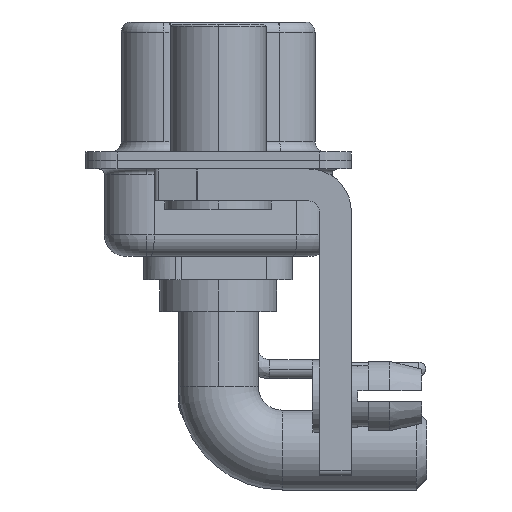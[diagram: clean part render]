
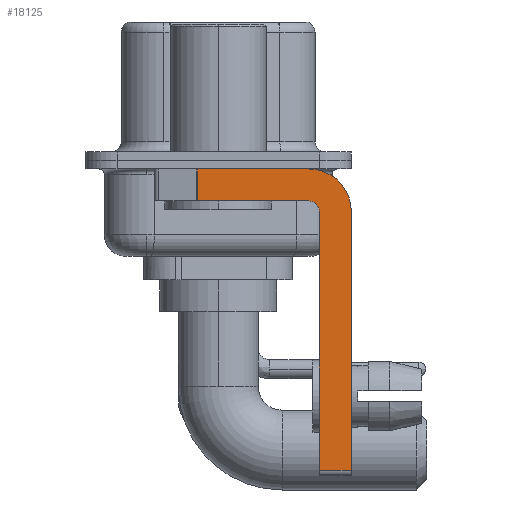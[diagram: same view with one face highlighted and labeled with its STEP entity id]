
A CAD part, left-side view. The second image highlights one B-rep face of the part: STEP entity #18125.
In plain terms, the highlighted planar face has unit normal (-1, 0, 0).
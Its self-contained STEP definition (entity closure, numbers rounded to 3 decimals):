
#287 = VERTEX_POINT ( 'NONE', #3551 ) ;
#379 = ORIENTED_EDGE ( 'NONE', *, *, #6843, .F. ) ;
#879 = DIRECTION ( 'NONE',  ( 0., 1., 0. ) ) ;
#1448 = EDGE_CURVE ( 'NONE', #28031, #14487, #7730, .T. ) ;
#1496 = CARTESIAN_POINT ( 'NONE',  ( -2.9, -4.25, -2.4 ) ) ;
#1642 = DIRECTION ( 'NONE',  ( 1., 0., 0. ) ) ;
#2060 = ORIENTED_EDGE ( 'NONE', *, *, #16158, .F. ) ;
#2559 = CARTESIAN_POINT ( 'NONE',  ( -2.9, 3., -0.4 ) ) ;
#3353 = EDGE_CURVE ( 'NONE', #16986, #287, #12311, .T. ) ;
#3551 = CARTESIAN_POINT ( 'NONE',  ( -2.9, -4.25, -1.9 ) ) ;
#4615 = VERTEX_POINT ( 'NONE', #22321 ) ;
#6075 = CARTESIAN_POINT ( 'NONE',  ( -2.9, -4.25, -0.4 ) ) ;
#6263 = LINE ( 'NONE', #14926, #11368 ) ;
#6843 = EDGE_CURVE ( 'NONE', #4615, #16986, #25310, .T. ) ;
#7092 = EDGE_CURVE ( 'NONE', #287, #12304, #11793, .T. ) ;
#7130 = CARTESIAN_POINT ( 'NONE',  ( -2.9, -4.25, -1.9 ) ) ;
#7249 = ORIENTED_EDGE ( 'NONE', *, *, #1448, .F. ) ;
#7374 = CARTESIAN_POINT ( 'NONE',  ( -2.9, -6.25, -2.4 ) ) ;
#7390 = CARTESIAN_POINT ( 'NONE',  ( -2.9, -4.25, -2.4 ) ) ;
#7487 = VECTOR ( 'NONE', #20185, 1000. ) ;
#7683 = VECTOR ( 'NONE', #21189, 1000. ) ;
#7730 = CIRCLE ( 'NONE', #23120, 2. ) ;
#7964 = DIRECTION ( 'NONE',  ( 0., 0., -1. ) ) ;
#8026 = DIRECTION ( 'NONE',  ( 0., 0., -1. ) ) ;
#8155 = ORIENTED_EDGE ( 'NONE', *, *, #24851, .F. ) ;
#8399 = DIRECTION ( 'NONE',  ( -1., 0., 0. ) ) ;
#9856 = EDGE_CURVE ( 'NONE', #27472, #12304, #6263, .T. ) ;
#11368 = VECTOR ( 'NONE', #7964, 1000. ) ;
#11793 = LINE ( 'NONE', #7130, #19446 ) ;
#12195 = LINE ( 'NONE', #7374, #16319 ) ;
#12304 = VERTEX_POINT ( 'NONE', #23825 ) ;
#12311 = CIRCLE ( 'NONE', #25896, 0.5 ) ;
#13154 = ORIENTED_EDGE ( 'NONE', *, *, #9856, .T. ) ;
#13364 = ORIENTED_EDGE ( 'NONE', *, *, #18329, .T. ) ;
#13800 = CARTESIAN_POINT ( 'NONE',  ( -2.9, -6.25, -2.4 ) ) ;
#13816 = CARTESIAN_POINT ( 'NONE',  ( -2.9, -4.25, -14.55 ) ) ;
#14419 = FACE_OUTER_BOUND ( 'NONE', #21427, .T. ) ;
#14487 = VERTEX_POINT ( 'NONE', #13800 ) ;
#14926 = CARTESIAN_POINT ( 'NONE',  ( -2.9, 0.978, -1.9 ) ) ;
#15188 = LINE ( 'NONE', #2559, #20633 ) ;
#16158 = EDGE_CURVE ( 'NONE', #27472, #28031, #15188, .T. ) ;
#16173 = CARTESIAN_POINT ( 'NONE',  ( -2.9, -6.25, -14.55 ) ) ;
#16319 = VECTOR ( 'NONE', #20415, 1000. ) ;
#16986 = VERTEX_POINT ( 'NONE', #25186 ) ;
#17198 = CARTESIAN_POINT ( 'NONE',  ( -2.9, -4.25, -2.4 ) ) ;
#18125 = ADVANCED_FACE ( 'NONE', ( #14419 ), #27313, .F. ) ;
#18329 = EDGE_CURVE ( 'NONE', #4615, #24887, #22036, .T. ) ;
#18885 = DIRECTION ( 'NONE',  ( 0., 0., 1. ) ) ;
#19446 = VECTOR ( 'NONE', #879, 1000. ) ;
#19543 = ORIENTED_EDGE ( 'NONE', *, *, #7092, .F. ) ;
#20011 = DIRECTION ( 'NONE',  ( 1., 0., 0. ) ) ;
#20185 = DIRECTION ( 'NONE',  ( 0., -1., 0. ) ) ;
#20411 = ORIENTED_EDGE ( 'NONE', *, *, #3353, .F. ) ;
#20415 = DIRECTION ( 'NONE',  ( 0., 0., -1. ) ) ;
#20633 = VECTOR ( 'NONE', #21700, 1000. ) ;
#21189 = DIRECTION ( 'NONE',  ( 0., 0., 1. ) ) ;
#21427 = EDGE_LOOP ( 'NONE', ( #2060, #13154, #19543, #20411, #379, #13364, #8155, #7249 ) ) ;
#21700 = DIRECTION ( 'NONE',  ( 0., -1., 0. ) ) ;
#22036 = LINE ( 'NONE', #13816, #7487 ) ;
#22321 = CARTESIAN_POINT ( 'NONE',  ( -2.9, -4.75, -14.55 ) ) ;
#23120 = AXIS2_PLACEMENT_3D ( 'NONE', #7390, #20011, #24289 ) ;
#23825 = CARTESIAN_POINT ( 'NONE',  ( -2.9, 0.978, -1.9 ) ) ;
#24289 = DIRECTION ( 'NONE',  ( 0., 0., -1. ) ) ;
#24729 = CARTESIAN_POINT ( 'NONE',  ( -2.9, 0.978, -0.4 ) ) ;
#24851 = EDGE_CURVE ( 'NONE', #14487, #24887, #12195, .T. ) ;
#24887 = VERTEX_POINT ( 'NONE', #16173 ) ;
#25033 = CARTESIAN_POINT ( 'NONE',  ( -2.9, -4.75, -14.8 ) ) ;
#25186 = CARTESIAN_POINT ( 'NONE',  ( -2.9, -4.75, -2.4 ) ) ;
#25310 = LINE ( 'NONE', #25033, #7683 ) ;
#25896 = AXIS2_PLACEMENT_3D ( 'NONE', #17198, #8399, #18885 ) ;
#27313 = PLANE ( 'NONE',  #27861 ) ;
#27472 = VERTEX_POINT ( 'NONE', #24729 ) ;
#27861 = AXIS2_PLACEMENT_3D ( 'NONE', #1496, #1642, #8026 ) ;
#28031 = VERTEX_POINT ( 'NONE', #6075 ) ;
